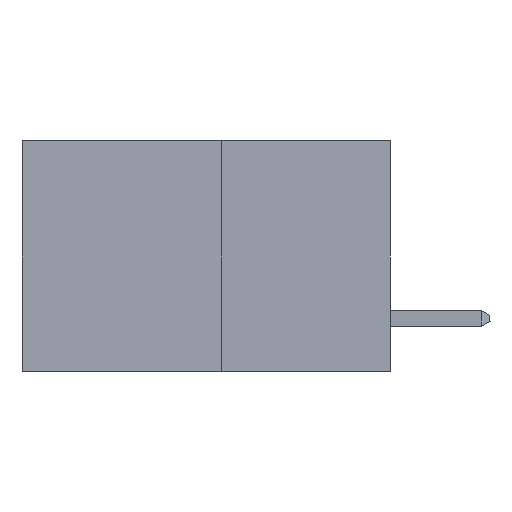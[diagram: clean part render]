
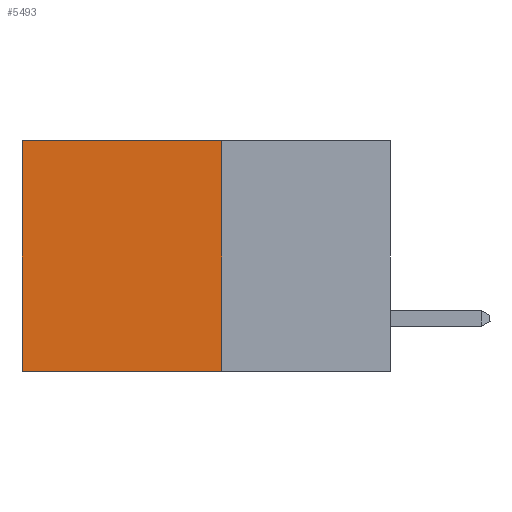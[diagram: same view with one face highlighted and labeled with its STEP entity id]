
A CAD part, left-side view. The second image highlights one B-rep face of the part: STEP entity #5493.
In plain terms, the highlighted planar face has unit normal (-1, 0, 0).
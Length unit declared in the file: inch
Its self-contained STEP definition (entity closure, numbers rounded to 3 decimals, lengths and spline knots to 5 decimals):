
#114 = VERTEX_POINT ( 'NONE', #6792 ) ;
#386 = VECTOR ( 'NONE', #4727, 39.37008 ) ;
#507 = CARTESIAN_POINT ( 'NONE',  ( 0.277, 0.27, -0.37 ) ) ;
#526 = VECTOR ( 'NONE', #1097, 39.37008 ) ;
#989 = ORIENTED_EDGE ( 'NONE', *, *, #5356, .F. ) ;
#991 = DIRECTION ( 'NONE',  ( 0., 1., 0. ) ) ;
#1097 = DIRECTION ( 'NONE',  ( 0., 1., 0. ) ) ;
#1290 = CARTESIAN_POINT ( 'NONE',  ( 0.277, 0.27, 0. ) ) ;
#1358 = VERTEX_POINT ( 'NONE', #1290 ) ;
#1429 = CARTESIAN_POINT ( 'NONE',  ( 0.277, 0.59, 0. ) ) ;
#2470 = FACE_OUTER_BOUND ( 'NONE', #3205, .T. ) ;
#2537 = LINE ( 'NONE', #2687, #4873 ) ;
#2687 = CARTESIAN_POINT ( 'NONE',  ( 0.277, 0.27, 0. ) ) ;
#3205 = EDGE_LOOP ( 'NONE', ( #5364, #12080, #989, #6019 ) ) ;
#3264 = LINE ( 'NONE', #6103, #526 ) ;
#3332 = EDGE_CURVE ( 'NONE', #1358, #5110, #2537, .T. ) ;
#3719 = VECTOR ( 'NONE', #10780, 39.37008 ) ;
#4727 = DIRECTION ( 'NONE',  ( 0., 0., -1. ) ) ;
#4873 = VECTOR ( 'NONE', #991, 39.37008 ) ;
#5110 = VERTEX_POINT ( 'NONE', #1429 ) ;
#5356 = EDGE_CURVE ( 'NONE', #1358, #7650, #9350, .T. ) ;
#5364 = ORIENTED_EDGE ( 'NONE', *, *, #10941, .T. ) ;
#5493 = ADVANCED_FACE ( 'NONE', ( #2470 ), #12034, .F. ) ;
#6019 = ORIENTED_EDGE ( 'NONE', *, *, #3332, .T. ) ;
#6103 = CARTESIAN_POINT ( 'NONE',  ( 0.277, 0.27, -0.37 ) ) ;
#6754 = AXIS2_PLACEMENT_3D ( 'NONE', #11710, #11665, #11682 ) ;
#6759 = CARTESIAN_POINT ( 'NONE',  ( 0.277, 0.59, -0.37 ) ) ;
#6792 = CARTESIAN_POINT ( 'NONE',  ( 0.277, 0.59, -0.37 ) ) ;
#7650 = VERTEX_POINT ( 'NONE', #507 ) ;
#8442 = LINE ( 'NONE', #6759, #386 ) ;
#9350 = LINE ( 'NONE', #10519, #3719 ) ;
#10519 = CARTESIAN_POINT ( 'NONE',  ( 0.277, 0.27, -0.37 ) ) ;
#10780 = DIRECTION ( 'NONE',  ( 0., 0., -1. ) ) ;
#10941 = EDGE_CURVE ( 'NONE', #5110, #114, #8442, .T. ) ;
#11665 = DIRECTION ( 'NONE',  ( 1., 0., 0. ) ) ;
#11682 = DIRECTION ( 'NONE',  ( 0., 0., -1. ) ) ;
#11710 = CARTESIAN_POINT ( 'NONE',  ( 0.277, 0.27, -0.37 ) ) ;
#12034 = PLANE ( 'NONE',  #6754 ) ;
#12080 = ORIENTED_EDGE ( 'NONE', *, *, #12465, .F. ) ;
#12465 = EDGE_CURVE ( 'NONE', #7650, #114, #3264, .T. ) ;
